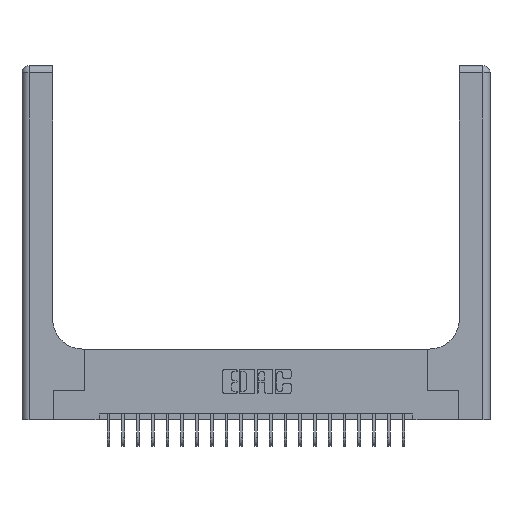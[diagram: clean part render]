
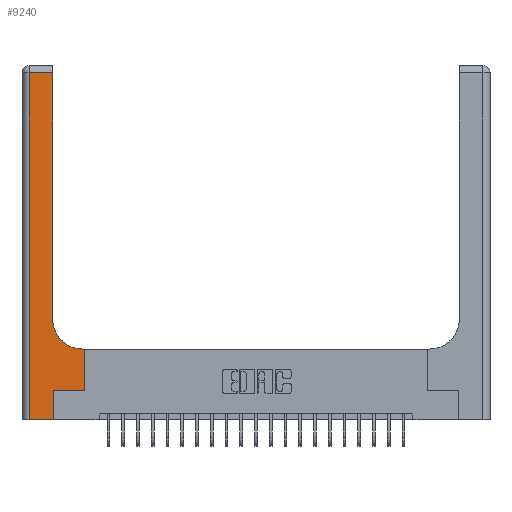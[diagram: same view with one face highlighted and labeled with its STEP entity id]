
A CAD part, top view. The second image highlights one B-rep face of the part: STEP entity #9240.
In plain terms, the highlighted planar face has unit normal (0, 0, 1).
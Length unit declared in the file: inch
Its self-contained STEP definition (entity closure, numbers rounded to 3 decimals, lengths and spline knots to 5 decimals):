
#48 = VECTOR ( 'NONE', #2191, 39.37008 ) ;
#220 = ORIENTED_EDGE ( 'NONE', *, *, #23450, .T. ) ;
#263 = VECTOR ( 'NONE', #6546, 39.37008 ) ;
#762 = VERTEX_POINT ( 'NONE', #21128 ) ;
#780 = EDGE_LOOP ( 'NONE', ( #10905, #18963, #6324, #8565, #16048, #10279, #17729, #21963, #220 ) ) ;
#866 = VECTOR ( 'NONE', #20361, 39.37008 ) ;
#961 = DIRECTION ( 'NONE',  ( 0., -1., 0. ) ) ;
#1084 = LINE ( 'NONE', #12101, #10631 ) ;
#1474 = CARTESIAN_POINT ( 'NONE',  ( 0.26, 0.6, 0.37 ) ) ;
#2191 = DIRECTION ( 'NONE',  ( 0., 1., 0. ) ) ;
#2203 = VERTEX_POINT ( 'NONE', #4221 ) ;
#2205 = VERTEX_POINT ( 'NONE', #12642 ) ;
#2887 = PLANE ( 'NONE',  #9414 ) ;
#4221 = CARTESIAN_POINT ( 'NONE',  ( 0.265, 0.25, 0.37 ) ) ;
#5032 = EDGE_CURVE ( 'NONE', #8412, #9541, #8244, .T. ) ;
#5087 = VECTOR ( 'NONE', #10574, 39.37008 ) ;
#5886 = DIRECTION ( 'NONE',  ( 1., 0., 0. ) ) ;
#6324 = ORIENTED_EDGE ( 'NONE', *, *, #22731, .T. ) ;
#6364 = DIRECTION ( 'NONE',  ( 0., 0., -1. ) ) ;
#6546 = DIRECTION ( 'NONE',  ( 0., 1., 0. ) ) ;
#6778 = CARTESIAN_POINT ( 'NONE',  ( 0.06, 0., 0.37 ) ) ;
#6843 = DIRECTION ( 'NONE',  ( 1., 0., 0. ) ) ;
#6900 = CARTESIAN_POINT ( 'NONE',  ( 0.265, 0., 0.37 ) ) ;
#7351 = EDGE_CURVE ( 'NONE', #8123, #762, #20403, .T. ) ;
#8123 = VERTEX_POINT ( 'NONE', #23134 ) ;
#8244 = LINE ( 'NONE', #19278, #48 ) ;
#8383 = EDGE_CURVE ( 'NONE', #13433, #2205, #18050, .T. ) ;
#8412 = VERTEX_POINT ( 'NONE', #10639 ) ;
#8565 = ORIENTED_EDGE ( 'NONE', *, *, #8383, .T. ) ;
#8864 = DIRECTION ( 'NONE',  ( -1., 0., 0. ) ) ;
#9066 = CARTESIAN_POINT ( 'NONE',  ( 0., 0., 0.37 ) ) ;
#9168 = VERTEX_POINT ( 'NONE', #16369 ) ;
#9183 = VERTEX_POINT ( 'NONE', #11619 ) ;
#9204 = CARTESIAN_POINT ( 'NONE',  ( 0., 2.94, 0.37 ) ) ;
#9240 = ADVANCED_FACE ( 'NONE', ( #19150 ), #2887, .F. ) ;
#9414 = AXIS2_PLACEMENT_3D ( 'NONE', #17445, #10285, #21216 ) ;
#9496 = CIRCLE ( 'NONE', #16851, 0.25 ) ;
#9541 = VERTEX_POINT ( 'NONE', #9780 ) ;
#9780 = CARTESIAN_POINT ( 'NONE',  ( 0.528, 0.6, 0.37 ) ) ;
#10279 = ORIENTED_EDGE ( 'NONE', *, *, #23562, .T. ) ;
#10285 = DIRECTION ( 'NONE',  ( 0., 0., -1. ) ) ;
#10574 = DIRECTION ( 'NONE',  ( 0., 1., 0. ) ) ;
#10631 = VECTOR ( 'NONE', #961, 39.37008 ) ;
#10639 = CARTESIAN_POINT ( 'NONE',  ( 0.528, 0.25, 0.37 ) ) ;
#10905 = ORIENTED_EDGE ( 'NONE', *, *, #7351, .T. ) ;
#11619 = CARTESIAN_POINT ( 'NONE',  ( 0.06, 2.94, 0.37 ) ) ;
#12101 = CARTESIAN_POINT ( 'NONE',  ( 0.06, 3., 0.37 ) ) ;
#12482 = VECTOR ( 'NONE', #16457, 39.37008 ) ;
#12642 = CARTESIAN_POINT ( 'NONE',  ( 0.265, 0., 0.37 ) ) ;
#13084 = EDGE_CURVE ( 'NONE', #9541, #9168, #16378, .T. ) ;
#13433 = VERTEX_POINT ( 'NONE', #6778 ) ;
#14529 = VECTOR ( 'NONE', #6843, 39.37008 ) ;
#14896 = VECTOR ( 'NONE', #8864, 39.37008 ) ;
#15215 = EDGE_CURVE ( 'NONE', #2205, #2203, #23369, .T. ) ;
#16048 = ORIENTED_EDGE ( 'NONE', *, *, #15215, .T. ) ;
#16369 = CARTESIAN_POINT ( 'NONE',  ( 0.51, 0.6, 0.37 ) ) ;
#16378 = LINE ( 'NONE', #1474, #14896 ) ;
#16457 = DIRECTION ( 'NONE',  ( 1., 0., 0. ) ) ;
#16712 = LINE ( 'NONE', #9204, #866 ) ;
#16851 = AXIS2_PLACEMENT_3D ( 'NONE', #20917, #6364, #5886 ) ;
#17445 = CARTESIAN_POINT ( 'NONE',  ( 0., 3., 0.37 ) ) ;
#17729 = ORIENTED_EDGE ( 'NONE', *, *, #5032, .T. ) ;
#18018 = EDGE_CURVE ( 'NONE', #762, #9183, #16712, .T. ) ;
#18050 = LINE ( 'NONE', #9066, #12482 ) ;
#18963 = ORIENTED_EDGE ( 'NONE', *, *, #18018, .T. ) ;
#19150 = FACE_OUTER_BOUND ( 'NONE', #780, .T. ) ;
#19278 = CARTESIAN_POINT ( 'NONE',  ( 0.528, 0.25, 0.37 ) ) ;
#19809 = LINE ( 'NONE', #21631, #14529 ) ;
#20361 = DIRECTION ( 'NONE',  ( -1., 0., 0. ) ) ;
#20403 = LINE ( 'NONE', #22213, #5087 ) ;
#20917 = CARTESIAN_POINT ( 'NONE',  ( 0.51, 0.85, 0.37 ) ) ;
#21128 = CARTESIAN_POINT ( 'NONE',  ( 0.26, 2.94, 0.37 ) ) ;
#21216 = DIRECTION ( 'NONE',  ( -1., 0., 0. ) ) ;
#21631 = CARTESIAN_POINT ( 'NONE',  ( 0.265, 0.25, 0.37 ) ) ;
#21963 = ORIENTED_EDGE ( 'NONE', *, *, #13084, .T. ) ;
#22213 = CARTESIAN_POINT ( 'NONE',  ( 0.26, 3., 0.37 ) ) ;
#22731 = EDGE_CURVE ( 'NONE', #9183, #13433, #1084, .T. ) ;
#23134 = CARTESIAN_POINT ( 'NONE',  ( 0.26, 0.85, 0.37 ) ) ;
#23369 = LINE ( 'NONE', #6900, #263 ) ;
#23450 = EDGE_CURVE ( 'NONE', #9168, #8123, #9496, .T. ) ;
#23562 = EDGE_CURVE ( 'NONE', #2203, #8412, #19809, .T. ) ;
